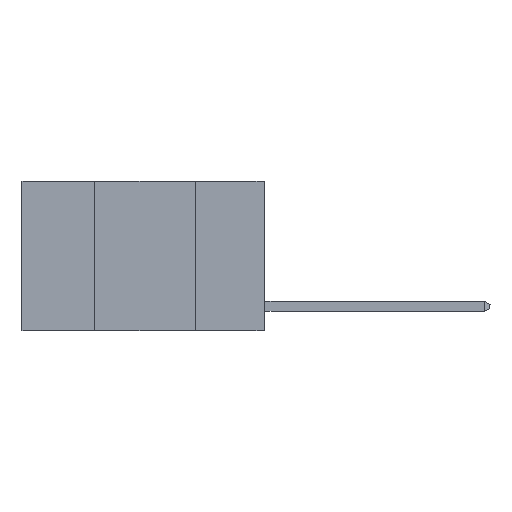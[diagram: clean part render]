
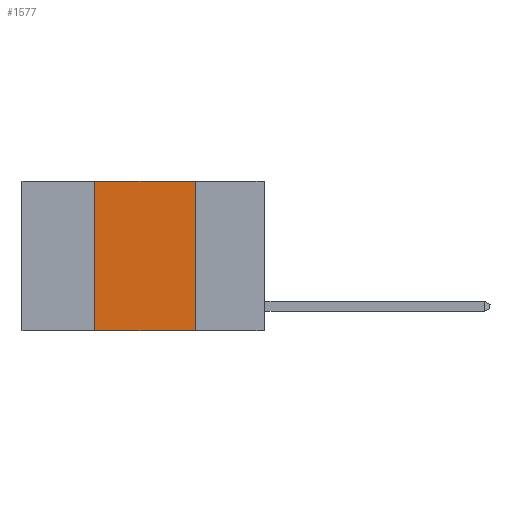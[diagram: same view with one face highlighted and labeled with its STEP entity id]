
A CAD part, left-side view. The second image highlights one B-rep face of the part: STEP entity #1577.
In plain terms, the highlighted planar face has unit normal (-1, 0, 0).
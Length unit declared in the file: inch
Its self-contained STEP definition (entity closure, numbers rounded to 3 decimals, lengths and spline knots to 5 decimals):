
#115 = FACE_OUTER_BOUND ( 'NONE', #1233, .T. ) ;
#598 = EDGE_CURVE ( 'NONE', #10309, #1540, #9439, .T. ) ;
#732 = VERTEX_POINT ( 'NONE', #3952 ) ;
#855 = CARTESIAN_POINT ( 'NONE',  ( 0., 0.17, -0.37 ) ) ;
#969 = CARTESIAN_POINT ( 'NONE',  ( 0., 0.6, -0.37 ) ) ;
#1233 = EDGE_LOOP ( 'NONE', ( #11809, #7392, #10068, #12675 ) ) ;
#1392 = DIRECTION ( 'NONE',  ( 0., -1., 0. ) ) ;
#1540 = VERTEX_POINT ( 'NONE', #855 ) ;
#1577 = ADVANCED_FACE ( 'NONE', ( #115 ), #10581, .F. ) ;
#2016 = VECTOR ( 'NONE', #9599, 39.37008 ) ;
#3397 = VECTOR ( 'NONE', #4687, 39.37008 ) ;
#3696 = VERTEX_POINT ( 'NONE', #6325 ) ;
#3952 = CARTESIAN_POINT ( 'NONE',  ( 0., 0.17, 0. ) ) ;
#4687 = DIRECTION ( 'NONE',  ( 0., 0., -1. ) ) ;
#5418 = EDGE_CURVE ( 'NONE', #10309, #3696, #7818, .T. ) ;
#5691 = EDGE_CURVE ( 'NONE', #732, #1540, #8756, .T. ) ;
#6325 = CARTESIAN_POINT ( 'NONE',  ( 0., 0.42, 0. ) ) ;
#7392 = ORIENTED_EDGE ( 'NONE', *, *, #10497, .F. ) ;
#7488 = VECTOR ( 'NONE', #8264, 39.37008 ) ;
#7633 = DIRECTION ( 'NONE',  ( 1., 0., 0. ) ) ;
#7818 = LINE ( 'NONE', #11217, #7488 ) ;
#8264 = DIRECTION ( 'NONE',  ( 0., 0., 1. ) ) ;
#8756 = LINE ( 'NONE', #9747, #3397 ) ;
#9439 = LINE ( 'NONE', #969, #2016 ) ;
#9580 = DIRECTION ( 'NONE',  ( 0., 0., -1. ) ) ;
#9599 = DIRECTION ( 'NONE',  ( 0., -1., 0. ) ) ;
#9747 = CARTESIAN_POINT ( 'NONE',  ( 0., 0.17, 0. ) ) ;
#10068 = ORIENTED_EDGE ( 'NONE', *, *, #5418, .F. ) ;
#10118 = CARTESIAN_POINT ( 'NONE',  ( 0., 0.6, 0. ) ) ;
#10125 = CARTESIAN_POINT ( 'NONE',  ( 0., 0.42, -0.37 ) ) ;
#10309 = VERTEX_POINT ( 'NONE', #10125 ) ;
#10374 = VECTOR ( 'NONE', #1392, 39.37008 ) ;
#10497 = EDGE_CURVE ( 'NONE', #3696, #732, #12944, .T. ) ;
#10581 = PLANE ( 'NONE',  #12358 ) ;
#11217 = CARTESIAN_POINT ( 'NONE',  ( 0., 0.42, 0. ) ) ;
#11492 = CARTESIAN_POINT ( 'NONE',  ( 0., 0.6, 0. ) ) ;
#11809 = ORIENTED_EDGE ( 'NONE', *, *, #5691, .F. ) ;
#12358 = AXIS2_PLACEMENT_3D ( 'NONE', #10118, #7633, #9580 ) ;
#12675 = ORIENTED_EDGE ( 'NONE', *, *, #598, .T. ) ;
#12944 = LINE ( 'NONE', #11492, #10374 ) ;
